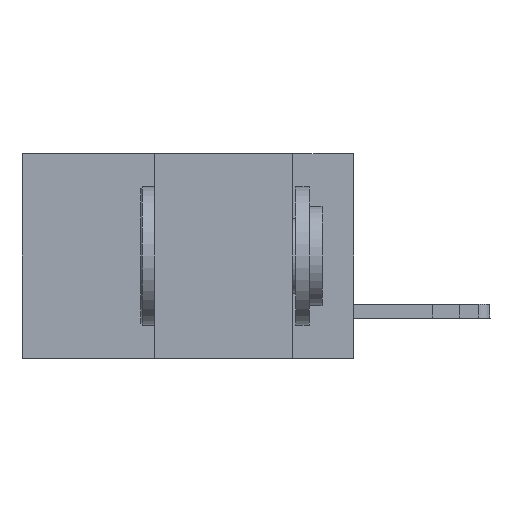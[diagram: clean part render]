
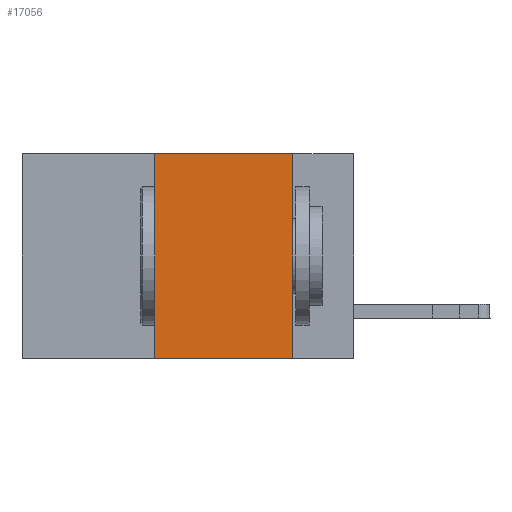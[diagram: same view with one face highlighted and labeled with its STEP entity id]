
A CAD part, left-side view. The second image highlights one B-rep face of the part: STEP entity #17056.
In plain terms, the highlighted planar face has unit normal (-1, 0, 0).
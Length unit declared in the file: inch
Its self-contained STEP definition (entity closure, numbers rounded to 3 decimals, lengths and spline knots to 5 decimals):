
#166 = FACE_OUTER_BOUND ( 'NONE', #5807, .T. ) ;
#1008 = EDGE_CURVE ( 'NONE', #4237, #11853, #17515, .T. ) ;
#1200 = LINE ( 'NONE', #14004, #6213 ) ;
#1282 = ORIENTED_EDGE ( 'NONE', *, *, #1008, .F. ) ;
#1647 = CARTESIAN_POINT ( 'NONE',  ( 0., 0.36, 0. ) ) ;
#2706 = ORIENTED_EDGE ( 'NONE', *, *, #15987, .F. ) ;
#3068 = DIRECTION ( 'NONE',  ( 0., 0., 1. ) ) ;
#4237 = VERTEX_POINT ( 'NONE', #22440 ) ;
#4325 = CARTESIAN_POINT ( 'NONE',  ( 0., 0.6, -0.37 ) ) ;
#4467 = CARTESIAN_POINT ( 'NONE',  ( 0., 0.11, -0.37 ) ) ;
#4691 = AXIS2_PLACEMENT_3D ( 'NONE', #17806, #5558, #12425 ) ;
#5558 = DIRECTION ( 'NONE',  ( 1., 0., 0. ) ) ;
#5807 = EDGE_LOOP ( 'NONE', ( #20680, #2706, #1282, #11379 ) ) ;
#5990 = CARTESIAN_POINT ( 'NONE',  ( 0., 0.36, 0. ) ) ;
#6076 = LINE ( 'NONE', #4325, #16261 ) ;
#6213 = VECTOR ( 'NONE', #22529, 39.37008 ) ;
#7924 = CARTESIAN_POINT ( 'NONE',  ( 0., 0.11, 0. ) ) ;
#10059 = CARTESIAN_POINT ( 'NONE',  ( 0., 0.11, 0. ) ) ;
#11379 = ORIENTED_EDGE ( 'NONE', *, *, #17642, .T. ) ;
#11853 = VERTEX_POINT ( 'NONE', #5990 ) ;
#12425 = DIRECTION ( 'NONE',  ( 0., 0., -1. ) ) ;
#14004 = CARTESIAN_POINT ( 'NONE',  ( 0., 0.6, 0. ) ) ;
#14239 = DIRECTION ( 'NONE',  ( 0., 0., -1. ) ) ;
#15851 = VERTEX_POINT ( 'NONE', #4467 ) ;
#15987 = EDGE_CURVE ( 'NONE', #11853, #22066, #1200, .T. ) ;
#16066 = EDGE_CURVE ( 'NONE', #22066, #15851, #18931, .T. ) ;
#16261 = VECTOR ( 'NONE', #20077, 39.37008 ) ;
#16652 = VECTOR ( 'NONE', #14239, 39.37008 ) ;
#17056 = ADVANCED_FACE ( 'NONE', ( #166 ), #22929, .F. ) ;
#17515 = LINE ( 'NONE', #1647, #20507 ) ;
#17642 = EDGE_CURVE ( 'NONE', #4237, #15851, #6076, .T. ) ;
#17806 = CARTESIAN_POINT ( 'NONE',  ( 0., 0.6, 0. ) ) ;
#18931 = LINE ( 'NONE', #10059, #16652 ) ;
#20077 = DIRECTION ( 'NONE',  ( 0., -1., 0. ) ) ;
#20507 = VECTOR ( 'NONE', #3068, 39.37008 ) ;
#20680 = ORIENTED_EDGE ( 'NONE', *, *, #16066, .F. ) ;
#22066 = VERTEX_POINT ( 'NONE', #7924 ) ;
#22440 = CARTESIAN_POINT ( 'NONE',  ( 0., 0.36, -0.37 ) ) ;
#22529 = DIRECTION ( 'NONE',  ( 0., -1., 0. ) ) ;
#22929 = PLANE ( 'NONE',  #4691 ) ;
